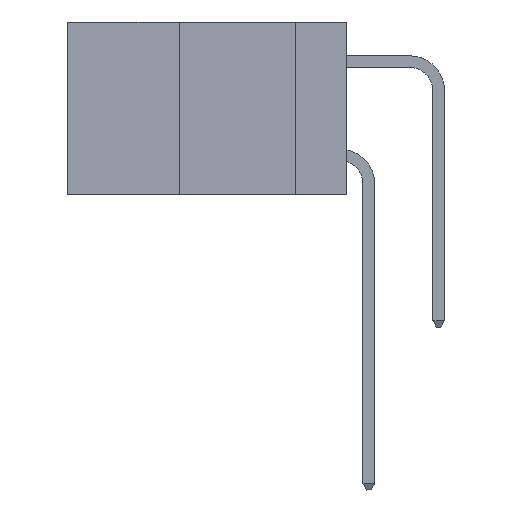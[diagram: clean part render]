
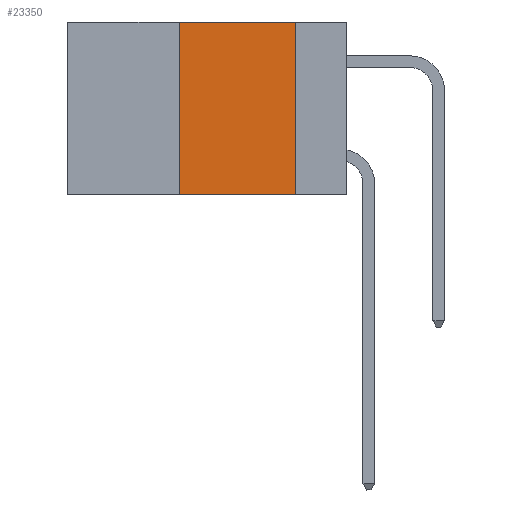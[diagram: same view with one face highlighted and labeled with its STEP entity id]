
A CAD part, left-side view. The second image highlights one B-rep face of the part: STEP entity #23350.
In plain terms, the highlighted planar face has unit normal (-1, 0, 0).
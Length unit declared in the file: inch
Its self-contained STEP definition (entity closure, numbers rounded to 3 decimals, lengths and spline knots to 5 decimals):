
#204 = VECTOR ( 'NONE', #7229, 39.37008 ) ;
#273 = VERTEX_POINT ( 'NONE', #18323 ) ;
#328 = CARTESIAN_POINT ( 'NONE',  ( 0., 0.36, 0. ) ) ;
#841 = DIRECTION ( 'NONE',  ( 1., 0., 0. ) ) ;
#1351 = CARTESIAN_POINT ( 'NONE',  ( 0., 0.11, -0.37 ) ) ;
#1372 = AXIS2_PLACEMENT_3D ( 'NONE', #10266, #841, #23080 ) ;
#2585 = EDGE_CURVE ( 'NONE', #273, #7575, #4369, .T. ) ;
#2715 = LINE ( 'NONE', #21687, #3872 ) ;
#2762 = VERTEX_POINT ( 'NONE', #328 ) ;
#3321 = CARTESIAN_POINT ( 'NONE',  ( 0., 0.36, 0. ) ) ;
#3333 = ORIENTED_EDGE ( 'NONE', *, *, #14561, .F. ) ;
#3872 = VECTOR ( 'NONE', #19833, 39.37008 ) ;
#4369 = LINE ( 'NONE', #16015, #23246 ) ;
#4622 = PLANE ( 'NONE',  #1372 ) ;
#6410 = VERTEX_POINT ( 'NONE', #6789 ) ;
#6789 = CARTESIAN_POINT ( 'NONE',  ( 0., 0.36, -0.37 ) ) ;
#7229 = DIRECTION ( 'NONE',  ( 0., 0., 1. ) ) ;
#7575 = VERTEX_POINT ( 'NONE', #1351 ) ;
#7655 = LINE ( 'NONE', #14677, #16238 ) ;
#8896 = EDGE_LOOP ( 'NONE', ( #23421, #14759, #3333, #13959 ) ) ;
#10266 = CARTESIAN_POINT ( 'NONE',  ( 0., 0.6, 0. ) ) ;
#12777 = LINE ( 'NONE', #3321, #204 ) ;
#13959 = ORIENTED_EDGE ( 'NONE', *, *, #20557, .T. ) ;
#14345 = DIRECTION ( 'NONE',  ( 0., 0., -1. ) ) ;
#14561 = EDGE_CURVE ( 'NONE', #6410, #2762, #12777, .T. ) ;
#14677 = CARTESIAN_POINT ( 'NONE',  ( 0., 0.6, -0.37 ) ) ;
#14759 = ORIENTED_EDGE ( 'NONE', *, *, #19710, .F. ) ;
#16015 = CARTESIAN_POINT ( 'NONE',  ( 0., 0.11, 0. ) ) ;
#16238 = VECTOR ( 'NONE', #18200, 39.37008 ) ;
#18200 = DIRECTION ( 'NONE',  ( 0., -1., 0. ) ) ;
#18323 = CARTESIAN_POINT ( 'NONE',  ( 0., 0.11, 0. ) ) ;
#19710 = EDGE_CURVE ( 'NONE', #2762, #273, #2715, .T. ) ;
#19833 = DIRECTION ( 'NONE',  ( 0., -1., 0. ) ) ;
#19989 = FACE_OUTER_BOUND ( 'NONE', #8896, .T. ) ;
#20557 = EDGE_CURVE ( 'NONE', #6410, #7575, #7655, .T. ) ;
#21687 = CARTESIAN_POINT ( 'NONE',  ( 0., 0.6, 0. ) ) ;
#23080 = DIRECTION ( 'NONE',  ( 0., 0., -1. ) ) ;
#23246 = VECTOR ( 'NONE', #14345, 39.37008 ) ;
#23350 = ADVANCED_FACE ( 'NONE', ( #19989 ), #4622, .F. ) ;
#23421 = ORIENTED_EDGE ( 'NONE', *, *, #2585, .F. ) ;
